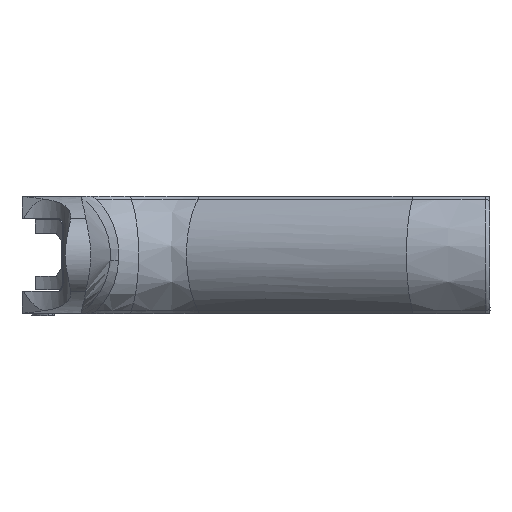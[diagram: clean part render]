
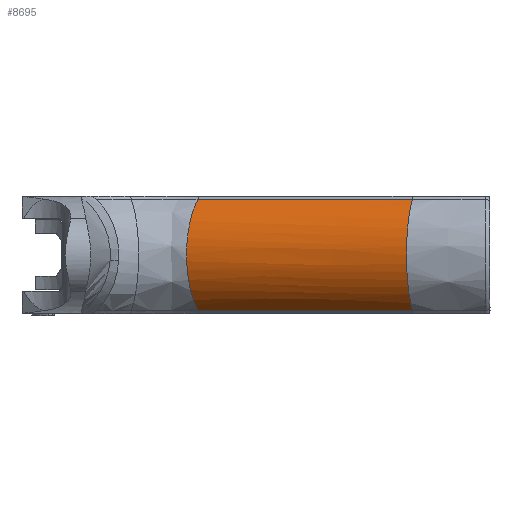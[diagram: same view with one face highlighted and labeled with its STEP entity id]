
A CAD part, left-side view. The second image highlights one B-rep face of the part: STEP entity #8695.
In plain terms, the highlighted free-form (B-spline) face has degree [3, 3] with [17, 4] control points.
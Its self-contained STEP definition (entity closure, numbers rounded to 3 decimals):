
#641=B_SPLINE_SURFACE_WITH_KNOTS('',3,3,((#13078,#13079,#13080,#13081),
(#13082,#13083,#13084,#13085),(#13086,#13087,#13088,#13089),(#13090,#13091,
#13092,#13093),(#13094,#13095,#13096,#13097),(#13098,#13099,#13100,#13101),
(#13102,#13103,#13104,#13105),(#13106,#13107,#13108,#13109),(#13110,#13111,
#13112,#13113),(#13114,#13115,#13116,#13117),(#13118,#13119,#13120,#13121),
(#13122,#13123,#13124,#13125),(#13126,#13127,#13128,#13129),(#13130,#13131,
#13132,#13133),(#13134,#13135,#13136,#13137),(#13138,#13139,#13140,#13141),
(#13142,#13143,#13144,#13145)),.UNSPECIFIED.,.F.,.F.,.F.,(4,1,1,1,1,1,1,
1,1,1,1,1,1,1,4),(4,4),(0.,0.124,0.165,0.238,
0.305,0.372,0.413,0.546,
0.579,0.613,0.679,0.752,
0.814,0.876,1.),(0.,1.),.UNSPECIFIED.);
#768=FACE_OUTER_BOUND('',#1262,.T.);
#1262=EDGE_LOOP('',(#5817,#5818,#5819,#5820));
#1749=B_SPLINE_CURVE_WITH_KNOTS('',3,(#12836,#12837,#12838,#12839,#12840,
#12841,#12842,#12843,#12844,#12845,#12846,#12847),.UNSPECIFIED.,.F.,.F.,
(4,2,2,2,2,4),(-3.581,-2.82,-2.054,-1.281,
-0.601,0.),.UNSPECIFIED.);
#1754=B_SPLINE_CURVE_WITH_KNOTS('',3,(#13052,#13053,#13054,#13055,#13056,
#13057,#13058,#13059,#13060,#13061,#13062,#13063),.UNSPECIFIED.,.F.,.F.,
(4,2,2,2,2,4),(-3.496,-2.782,-2.219,-1.418,
-0.614,0.),.UNSPECIFIED.);
#2008=LINE('',#12382,#2718);
#2054=LINE('',#13146,#2764);
#2718=VECTOR('',#9967,51.832);
#2764=VECTOR('',#10069,51.832);
#3429=VERTEX_POINT('',#12335);
#3432=VERTEX_POINT('',#12381);
#3479=VERTEX_POINT('',#12835);
#3485=VERTEX_POINT('',#13051);
#4321=EDGE_CURVE('',#3429,#3432,#2008,.T.);
#4381=EDGE_CURVE('',#3479,#3432,#1749,.T.);
#4396=EDGE_CURVE('',#3429,#3485,#1754,.T.);
#4399=EDGE_CURVE('',#3485,#3479,#2054,.T.);
#5817=ORIENTED_EDGE('',*,*,#4396,.T.);
#5818=ORIENTED_EDGE('',*,*,#4399,.T.);
#5819=ORIENTED_EDGE('',*,*,#4381,.T.);
#5820=ORIENTED_EDGE('',*,*,#4321,.F.);
#8695=ADVANCED_FACE('',(#768),#641,.T.);
#9967=DIRECTION('',(-0.313,-0.95,0.));
#10069=DIRECTION('',(-0.313,-0.95,0.));
#12335=CARTESIAN_POINT('',(-81.613,-31.44,-87.25));
#12381=CARTESIAN_POINT('',(-97.827,-80.67,-87.25));
#12382=CARTESIAN_POINT('',(-81.613,-31.44,-87.25));
#12835=CARTESIAN_POINT('',(-97.827,-80.67,-112.75));
#12836=CARTESIAN_POINT('Ctrl Pts',(-97.827,-80.67,
-112.75));
#12837=CARTESIAN_POINT('Ctrl Pts',(-99.295,-80.355,-111.635));
#12838=CARTESIAN_POINT('Ctrl Pts',(-100.565,-80.082,
-110.248));
#12839=CARTESIAN_POINT('Ctrl Pts',(-102.573,-79.651,
-107.108));
#12840=CARTESIAN_POINT('Ctrl Pts',(-103.29,-79.497,
-105.381));
#12841=CARTESIAN_POINT('Ctrl Pts',(-104.111,-79.321,
-101.694));
#12842=CARTESIAN_POINT('Ctrl Pts',(-104.233,-79.294,-99.627));
#12843=CARTESIAN_POINT('Ctrl Pts',(-103.601,-79.43,
-95.588));
#12844=CARTESIAN_POINT('Ctrl Pts',(-102.939,-79.572,
-93.582));
#12845=CARTESIAN_POINT('Ctrl Pts',(-100.741,-80.044,
-89.95));
#12846=CARTESIAN_POINT('Ctrl Pts',(-99.399,-80.333,-88.445));
#12847=CARTESIAN_POINT('Ctrl Pts',(-97.827,-80.67,-87.25));
#13051=CARTESIAN_POINT('',(-81.613,-31.44,-112.75));
#13052=CARTESIAN_POINT('Ctrl Pts',(-81.613,-31.44,
-87.25));
#13053=CARTESIAN_POINT('Ctrl Pts',(-82.574,-31.012,
-88.023));
#13054=CARTESIAN_POINT('Ctrl Pts',(-83.915,-30.414,
-89.288));
#13055=CARTESIAN_POINT('Ctrl Pts',(-86.053,-29.462,-92.793));
#13056=CARTESIAN_POINT('Ctrl Pts',(-86.749,-29.152,-94.522));
#13057=CARTESIAN_POINT('Ctrl Pts',(-87.722,-28.719,-98.897));
#13058=CARTESIAN_POINT('Ctrl Pts',(-87.574,-28.784,
-101.054));
#13059=CARTESIAN_POINT('Ctrl Pts',(-87.163,-28.968,
-103.876));
#13060=CARTESIAN_POINT('Ctrl Pts',(-86.684,-29.181,
-105.989));
#13061=CARTESIAN_POINT('Ctrl Pts',(-84.409,-30.194,
-110.006));
#13062=CARTESIAN_POINT('Ctrl Pts',(-83.12,-30.769,
-111.538));
#13063=CARTESIAN_POINT('Ctrl Pts',(-81.613,-31.44,-112.75));
#13078=CARTESIAN_POINT('Ctrl Pts',(-81.613,-31.44,
-87.25));
#13079=CARTESIAN_POINT('Ctrl Pts',(-87.018,-47.85,
-87.25));
#13080=CARTESIAN_POINT('Ctrl Pts',(-92.422,-64.26,
-87.25));
#13081=CARTESIAN_POINT('Ctrl Pts',(-97.827,-80.67,
-87.25));
#13082=CARTESIAN_POINT('Ctrl Pts',(-82.195,-31.181,
-87.718));
#13083=CARTESIAN_POINT('Ctrl Pts',(-87.793,-47.594,-87.858));
#13084=CARTESIAN_POINT('Ctrl Pts',(-93.387,-64.008,
-87.99));
#13085=CARTESIAN_POINT('Ctrl Pts',(-98.985,-80.421,
-88.13));
#13086=CARTESIAN_POINT('Ctrl Pts',(-83.157,-30.752,
-88.593));
#13087=CARTESIAN_POINT('Ctrl Pts',(-88.891,-47.21,
-88.903));
#13088=CARTESIAN_POINT('Ctrl Pts',(-94.624,-63.669,
-89.21));
#13089=CARTESIAN_POINT('Ctrl Pts',(-100.358,-80.127,
-89.52));
#13090=CARTESIAN_POINT('Ctrl Pts',(-84.605,-30.107,-90.406));
#13091=CARTESIAN_POINT('Ctrl Pts',(-90.389,-46.666,
-90.897));
#13092=CARTESIAN_POINT('Ctrl Pts',(-96.172,-63.225,-91.385));
#13093=CARTESIAN_POINT('Ctrl Pts',(-101.955,-79.784,
-91.876));
#13094=CARTESIAN_POINT('Ctrl Pts',(-85.697,-29.621,
-92.166));
#13095=CARTESIAN_POINT('Ctrl Pts',(-91.433,-46.274,
-92.695));
#13096=CARTESIAN_POINT('Ctrl Pts',(-97.169,-62.927,
-93.225));
#13097=CARTESIAN_POINT('Ctrl Pts',(-102.905,-79.58,
-93.755));
#13098=CARTESIAN_POINT('Ctrl Pts',(-86.624,-29.208,
-94.311));
#13099=CARTESIAN_POINT('Ctrl Pts',(-92.287,-45.948,
-94.836));
#13100=CARTESIAN_POINT('Ctrl Pts',(-97.949,-62.688,
-95.362));
#13101=CARTESIAN_POINT('Ctrl Pts',(-103.611,-79.428,
-95.888));
#13102=CARTESIAN_POINT('Ctrl Pts',(-87.176,-28.962,
-96.277));
#13103=CARTESIAN_POINT('Ctrl Pts',(-92.768,-45.76,
-96.736));
#13104=CARTESIAN_POINT('Ctrl Pts',(-98.359,-62.557,
-97.195));
#13105=CARTESIAN_POINT('Ctrl Pts',(-103.952,-79.355,
-97.654));
#13106=CARTESIAN_POINT('Ctrl Pts',(-87.602,-28.772,
-98.902));
#13107=CARTESIAN_POINT('Ctrl Pts',(-93.123,-45.618,
-99.274));
#13108=CARTESIAN_POINT('Ctrl Pts',(-98.643,-62.464,
-99.647));
#13109=CARTESIAN_POINT('Ctrl Pts',(-104.163,-79.309,
-100.02));
#13110=CARTESIAN_POINT('Ctrl Pts',(-87.565,-28.789,
-100.792));
#13111=CARTESIAN_POINT('Ctrl Pts',(-93.052,-45.639,
-101.188));
#13112=CARTESIAN_POINT('Ctrl Pts',(-98.538,-62.489,
-101.579));
#13113=CARTESIAN_POINT('Ctrl Pts',(-104.025,-79.339,
-101.975));
#13114=CARTESIAN_POINT('Ctrl Pts',(-87.41,-28.858,
-102.194));
#13115=CARTESIAN_POINT('Ctrl Pts',(-92.83,-45.71,
-102.696));
#13116=CARTESIAN_POINT('Ctrl Pts',(-98.251,-62.563,
-103.199));
#13117=CARTESIAN_POINT('Ctrl Pts',(-103.672,-79.415,
-103.7));
#13118=CARTESIAN_POINT('Ctrl Pts',(-87.292,-28.91,
-102.995));
#13119=CARTESIAN_POINT('Ctrl Pts',(-92.654,-45.766,
-103.606));
#13120=CARTESIAN_POINT('Ctrl Pts',(-98.016,-62.622,
-104.214));
#13121=CARTESIAN_POINT('Ctrl Pts',(-103.378,-79.478,-104.824));
#13122=CARTESIAN_POINT('Ctrl Pts',(-87.029,-29.027,
-104.296));
#13123=CARTESIAN_POINT('Ctrl Pts',(-92.314,-45.88,
-104.945));
#13124=CARTESIAN_POINT('Ctrl Pts',(-97.598,-62.732,-105.593));
#13125=CARTESIAN_POINT('Ctrl Pts',(-102.883,-79.584,
-106.242));
#13126=CARTESIAN_POINT('Ctrl Pts',(-86.486,-29.269,
-106.04));
#13127=CARTESIAN_POINT('Ctrl Pts',(-91.697,-46.096,
-106.632));
#13128=CARTESIAN_POINT('Ctrl Pts',(-96.909,-62.922,
-107.222));
#13129=CARTESIAN_POINT('Ctrl Pts',(-102.121,-79.748,
-107.815));
#13130=CARTESIAN_POINT('Ctrl Pts',(-85.618,-29.656,
-107.955));
#13131=CARTESIAN_POINT('Ctrl Pts',(-90.813,-46.419,
-108.394));
#13132=CARTESIAN_POINT('Ctrl Pts',(-96.008,-63.182,
-108.835));
#13133=CARTESIAN_POINT('Ctrl Pts',(-101.203,-79.945,
-109.274));
#13134=CARTESIAN_POINT('Ctrl Pts',(-84.103,-30.33,
-110.387));
#13135=CARTESIAN_POINT('Ctrl Pts',(-89.358,-46.964,
-110.586));
#13136=CARTESIAN_POINT('Ctrl Pts',(-94.613,-63.598,
-110.784));
#13137=CARTESIAN_POINT('Ctrl Pts',(-99.868,-80.232,
-110.983));
#13138=CARTESIAN_POINT('Ctrl Pts',(-82.678,-30.965,
-111.893));
#13139=CARTESIAN_POINT('Ctrl Pts',(-88.012,-47.473,-111.965));
#13140=CARTESIAN_POINT('Ctrl Pts',(-93.35,-63.979,
-112.027));
#13141=CARTESIAN_POINT('Ctrl Pts',(-98.684,-80.486,
-112.099));
#13142=CARTESIAN_POINT('Ctrl Pts',(-81.613,-31.44,
-112.75));
#13143=CARTESIAN_POINT('Ctrl Pts',(-87.018,-47.85,-112.75));
#13144=CARTESIAN_POINT('Ctrl Pts',(-92.422,-64.26,
-112.75));
#13145=CARTESIAN_POINT('Ctrl Pts',(-97.827,-80.67,
-112.75));
#13146=CARTESIAN_POINT('',(-81.613,-31.44,-112.75));
